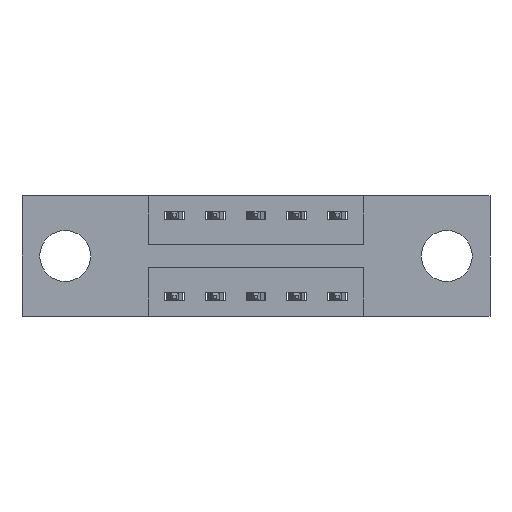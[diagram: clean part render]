
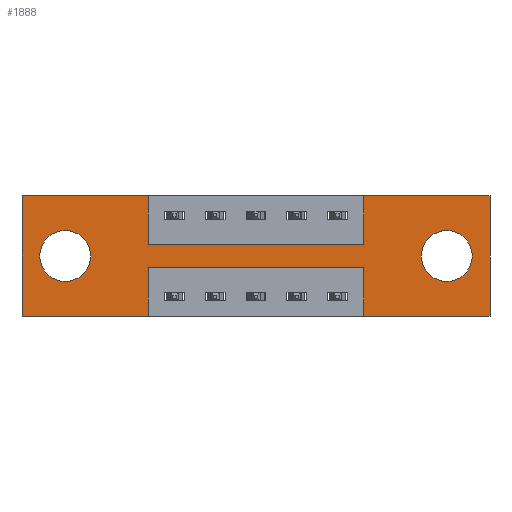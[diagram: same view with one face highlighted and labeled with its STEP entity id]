
A CAD part, front view. The second image highlights one B-rep face of the part: STEP entity #1888.
In plain terms, the highlighted planar face has unit normal (0, -1, 0).
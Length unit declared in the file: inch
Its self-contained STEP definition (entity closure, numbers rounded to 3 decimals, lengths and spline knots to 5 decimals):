
#2 = LINE ( 'NONE', #5316, #4423 ) ;
#27 = DIRECTION ( 'NONE',  ( 0., 0., 1. ) ) ;
#173 = CARTESIAN_POINT ( 'NONE',  ( 0.1325, 0., -0.185 ) ) ;
#321 = CARTESIAN_POINT ( 'NONE',  ( 1.435, 0., 0. ) ) ;
#589 = DIRECTION ( 'NONE',  ( 0., 0., -1. ) ) ;
#593 = DIRECTION ( 'NONE',  ( 1., 0., 0. ) ) ;
#650 = CARTESIAN_POINT ( 'NONE',  ( 0.3875, 0., -0.22 ) ) ;
#664 = CARTESIAN_POINT ( 'NONE',  ( 0.3875, 0., -0.22 ) ) ;
#682 = CARTESIAN_POINT ( 'NONE',  ( 0., 0., -0.37 ) ) ;
#709 = VERTEX_POINT ( 'NONE', #7439 ) ;
#757 = AXIS2_PLACEMENT_3D ( 'NONE', #7597, #4264, #6291 ) ;
#869 = ORIENTED_EDGE ( 'NONE', *, *, #1725, .F. ) ;
#896 = ORIENTED_EDGE ( 'NONE', *, *, #6861, .F. ) ;
#899 = CARTESIAN_POINT ( 'NONE',  ( 0., 0., -0.37 ) ) ;
#950 = VECTOR ( 'NONE', #1908, 39.37008 ) ;
#1017 = CARTESIAN_POINT ( 'NONE',  ( 0., 0., 0. ) ) ;
#1065 = EDGE_CURVE ( 'NONE', #4511, #2450, #3377, .T. ) ;
#1100 = CARTESIAN_POINT ( 'NONE',  ( 0., 0., -0.37 ) ) ;
#1180 = VERTEX_POINT ( 'NONE', #4470 ) ;
#1200 = EDGE_CURVE ( 'NONE', #3816, #7664, #7805, .T. ) ;
#1214 = EDGE_CURVE ( 'NONE', #2450, #1217, #8482, .T. ) ;
#1217 = VERTEX_POINT ( 'NONE', #1721 ) ;
#1367 = EDGE_CURVE ( 'NONE', #2865, #8260, #6062, .T. ) ;
#1375 = AXIS2_PLACEMENT_3D ( 'NONE', #173, #3599, #1462 ) ;
#1435 = EDGE_LOOP ( 'NONE', ( #1812, #5482 ) ) ;
#1462 = DIRECTION ( 'NONE',  ( 0., 0., 1. ) ) ;
#1578 = EDGE_CURVE ( 'NONE', #4732, #3952, #2862, .T. ) ;
#1675 = CARTESIAN_POINT ( 'NONE',  ( 1.0475, 0., -0.15 ) ) ;
#1693 = VERTEX_POINT ( 'NONE', #5274 ) ;
#1721 = CARTESIAN_POINT ( 'NONE',  ( 1.0475, 0., -0.22 ) ) ;
#1725 = EDGE_CURVE ( 'NONE', #5764, #3816, #2, .T. ) ;
#1812 = ORIENTED_EDGE ( 'NONE', *, *, #2716, .T. ) ;
#1823 = EDGE_LOOP ( 'NONE', ( #6298, #6415 ) ) ;
#1888 = ADVANCED_FACE ( 'NONE', ( #5363, #6755, #4700 ), #6717, .T. ) ;
#1905 = CARTESIAN_POINT ( 'NONE',  ( 0., 0., -0.37 ) ) ;
#1908 = DIRECTION ( 'NONE',  ( -1., 0., 0. ) ) ;
#2066 = ORIENTED_EDGE ( 'NONE', *, *, #5920, .F. ) ;
#2090 = CARTESIAN_POINT ( 'NONE',  ( 0.1325, 0., -0.185 ) ) ;
#2450 = VERTEX_POINT ( 'NONE', #4939 ) ;
#2476 = ORIENTED_EDGE ( 'NONE', *, *, #5136, .F. ) ;
#2652 = VECTOR ( 'NONE', #5933, 39.37008 ) ;
#2716 = EDGE_CURVE ( 'NONE', #8204, #4316, #2986, .T. ) ;
#2756 = DIRECTION ( 'NONE',  ( 0., 0., -1. ) ) ;
#2792 = ORIENTED_EDGE ( 'NONE', *, *, #5043, .F. ) ;
#2809 = ORIENTED_EDGE ( 'NONE', *, *, #1200, .F. ) ;
#2862 = CIRCLE ( 'NONE', #8066, 0.078 ) ;
#2865 = VERTEX_POINT ( 'NONE', #1675 ) ;
#2986 = CIRCLE ( 'NONE', #7922, 0.078 ) ;
#3231 = CARTESIAN_POINT ( 'NONE',  ( 1.3025, 0., -0.263 ) ) ;
#3239 = ORIENTED_EDGE ( 'NONE', *, *, #1065, .F. ) ;
#3300 = VECTOR ( 'NONE', #3335, 39.37008 ) ;
#3335 = DIRECTION ( 'NONE',  ( -1., 0., 0. ) ) ;
#3354 = VECTOR ( 'NONE', #5132, 39.37008 ) ;
#3377 = LINE ( 'NONE', #1905, #3300 ) ;
#3418 = ORIENTED_EDGE ( 'NONE', *, *, #5980, .F. ) ;
#3599 = DIRECTION ( 'NONE',  ( 0., 1., 0. ) ) ;
#3807 = CARTESIAN_POINT ( 'NONE',  ( 1.0475, 0., -0.37 ) ) ;
#3816 = VERTEX_POINT ( 'NONE', #1017 ) ;
#3838 = CARTESIAN_POINT ( 'NONE',  ( 1.3025, 0., -0.107 ) ) ;
#3843 = CARTESIAN_POINT ( 'NONE',  ( 0., 0., 0. ) ) ;
#3845 = LINE ( 'NONE', #321, #3354 ) ;
#3853 = CIRCLE ( 'NONE', #757, 0.078 ) ;
#3952 = VERTEX_POINT ( 'NONE', #4494 ) ;
#3989 = DIRECTION ( 'NONE',  ( 0., 1., 0. ) ) ;
#4032 = CARTESIAN_POINT ( 'NONE',  ( 1.3025, 0., -0.185 ) ) ;
#4255 = EDGE_CURVE ( 'NONE', #4316, #8204, #3853, .T. ) ;
#4264 = DIRECTION ( 'NONE',  ( 0., 1., 0. ) ) ;
#4316 = VERTEX_POINT ( 'NONE', #3231 ) ;
#4326 = VERTEX_POINT ( 'NONE', #664 ) ;
#4423 = VECTOR ( 'NONE', #7368, 39.37008 ) ;
#4470 = CARTESIAN_POINT ( 'NONE',  ( 0.3875, 0., -0.37 ) ) ;
#4494 = CARTESIAN_POINT ( 'NONE',  ( 0.1325, 0., -0.107 ) ) ;
#4511 = VERTEX_POINT ( 'NONE', #5747 ) ;
#4570 = ORIENTED_EDGE ( 'NONE', *, *, #1214, .F. ) ;
#4571 = VECTOR ( 'NONE', #6538, 39.37008 ) ;
#4700 = FACE_OUTER_BOUND ( 'NONE', #8543, .T. ) ;
#4729 = CARTESIAN_POINT ( 'NONE',  ( 1.0475, 0., 0. ) ) ;
#4732 = VERTEX_POINT ( 'NONE', #6068 ) ;
#4759 = LINE ( 'NONE', #650, #2652 ) ;
#4939 = CARTESIAN_POINT ( 'NONE',  ( 1.0475, 0., -0.37 ) ) ;
#5043 = EDGE_CURVE ( 'NONE', #1693, #4511, #3845, .T. ) ;
#5064 = DIRECTION ( 'NONE',  ( 0., 0., 1. ) ) ;
#5132 = DIRECTION ( 'NONE',  ( 0., 0., -1. ) ) ;
#5136 = EDGE_CURVE ( 'NONE', #4326, #1180, #7232, .T. ) ;
#5274 = CARTESIAN_POINT ( 'NONE',  ( 1.435, 0., 0. ) ) ;
#5316 = CARTESIAN_POINT ( 'NONE',  ( 0., 0., 0. ) ) ;
#5363 = FACE_BOUND ( 'NONE', #1435, .T. ) ;
#5398 = DIRECTION ( 'NONE',  ( 0., 0., -1. ) ) ;
#5482 = ORIENTED_EDGE ( 'NONE', *, *, #4255, .T. ) ;
#5510 = CARTESIAN_POINT ( 'NONE',  ( 0.3875, 0., -0.37 ) ) ;
#5592 = VECTOR ( 'NONE', #5838, 39.37008 ) ;
#5745 = ORIENTED_EDGE ( 'NONE', *, *, #1367, .F. ) ;
#5747 = CARTESIAN_POINT ( 'NONE',  ( 1.435, 0., -0.37 ) ) ;
#5748 = LINE ( 'NONE', #7713, #5592 ) ;
#5764 = VERTEX_POINT ( 'NONE', #899 ) ;
#5838 = DIRECTION ( 'NONE',  ( 1., 0., 0. ) ) ;
#5920 = EDGE_CURVE ( 'NONE', #1180, #5764, #8631, .T. ) ;
#5933 = DIRECTION ( 'NONE',  ( -1., 0., 0. ) ) ;
#5980 = EDGE_CURVE ( 'NONE', #7664, #709, #6636, .T. ) ;
#6062 = LINE ( 'NONE', #6572, #6146 ) ;
#6068 = CARTESIAN_POINT ( 'NONE',  ( 0.1325, 0., -0.263 ) ) ;
#6077 = DIRECTION ( 'NONE',  ( 0., -1., 0. ) ) ;
#6112 = AXIS2_PLACEMENT_3D ( 'NONE', #682, #6077, #5398 ) ;
#6146 = VECTOR ( 'NONE', #27, 39.37008 ) ;
#6183 = DIRECTION ( 'NONE',  ( 0., 0., -1. ) ) ;
#6291 = DIRECTION ( 'NONE',  ( 0., 0., -1. ) ) ;
#6298 = ORIENTED_EDGE ( 'NONE', *, *, #7188, .T. ) ;
#6395 = VECTOR ( 'NONE', #7721, 39.37008 ) ;
#6415 = ORIENTED_EDGE ( 'NONE', *, *, #1578, .T. ) ;
#6433 = ORIENTED_EDGE ( 'NONE', *, *, #7324, .F. ) ;
#6538 = DIRECTION ( 'NONE',  ( 1., 0., 0. ) ) ;
#6572 = CARTESIAN_POINT ( 'NONE',  ( 1.0475, 0., 0. ) ) ;
#6636 = LINE ( 'NONE', #6719, #8409 ) ;
#6715 = CIRCLE ( 'NONE', #1375, 0.078 ) ;
#6717 = PLANE ( 'NONE',  #6112 ) ;
#6719 = CARTESIAN_POINT ( 'NONE',  ( 0.3875, 0., 0. ) ) ;
#6755 = FACE_BOUND ( 'NONE', #1823, .T. ) ;
#6767 = ORIENTED_EDGE ( 'NONE', *, *, #8656, .F. ) ;
#6861 = EDGE_CURVE ( 'NONE', #8260, #1693, #5748, .T. ) ;
#7188 = EDGE_CURVE ( 'NONE', #3952, #4732, #6715, .T. ) ;
#7232 = LINE ( 'NONE', #5510, #8271 ) ;
#7291 = CARTESIAN_POINT ( 'NONE',  ( 0.3875, 0., -0.15 ) ) ;
#7324 = EDGE_CURVE ( 'NONE', #709, #2865, #8421, .T. ) ;
#7368 = DIRECTION ( 'NONE',  ( 0., 0., 1. ) ) ;
#7439 = CARTESIAN_POINT ( 'NONE',  ( 0.3875, 0., -0.15 ) ) ;
#7440 = DIRECTION ( 'NONE',  ( 0., 1., 0. ) ) ;
#7597 = CARTESIAN_POINT ( 'NONE',  ( 1.3025, 0., -0.185 ) ) ;
#7664 = VERTEX_POINT ( 'NONE', #8256 ) ;
#7713 = CARTESIAN_POINT ( 'NONE',  ( 0., 0., 0. ) ) ;
#7721 = DIRECTION ( 'NONE',  ( 0., 0., 1. ) ) ;
#7805 = LINE ( 'NONE', #3843, #4571 ) ;
#7838 = VECTOR ( 'NONE', #593, 39.37008 ) ;
#7922 = AXIS2_PLACEMENT_3D ( 'NONE', #4032, #3989, #589 ) ;
#8066 = AXIS2_PLACEMENT_3D ( 'NONE', #2090, #7440, #5064 ) ;
#8204 = VERTEX_POINT ( 'NONE', #3838 ) ;
#8256 = CARTESIAN_POINT ( 'NONE',  ( 0.3875, 0., 0. ) ) ;
#8260 = VERTEX_POINT ( 'NONE', #4729 ) ;
#8271 = VECTOR ( 'NONE', #6183, 39.37008 ) ;
#8409 = VECTOR ( 'NONE', #2756, 39.37008 ) ;
#8421 = LINE ( 'NONE', #7291, #7838 ) ;
#8482 = LINE ( 'NONE', #3807, #6395 ) ;
#8543 = EDGE_LOOP ( 'NONE', ( #2476, #6767, #4570, #3239, #2792, #896, #5745, #6433, #3418, #2809, #869, #2066 ) ) ;
#8631 = LINE ( 'NONE', #1100, #950 ) ;
#8656 = EDGE_CURVE ( 'NONE', #1217, #4326, #4759, .T. ) ;
